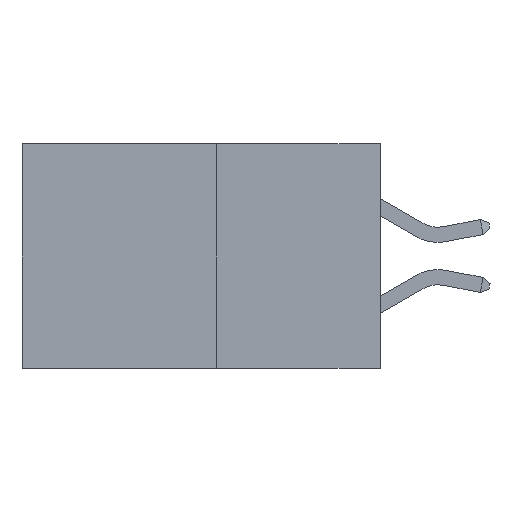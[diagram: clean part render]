
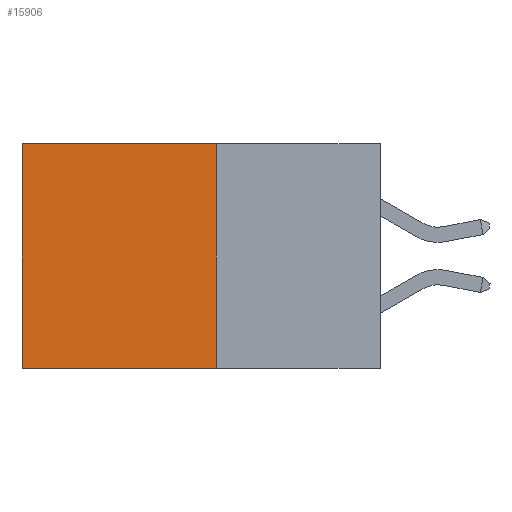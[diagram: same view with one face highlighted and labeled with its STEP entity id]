
A CAD part, left-side view. The second image highlights one B-rep face of the part: STEP entity #15906.
In plain terms, the highlighted planar face has unit normal (-1, 0, 0).
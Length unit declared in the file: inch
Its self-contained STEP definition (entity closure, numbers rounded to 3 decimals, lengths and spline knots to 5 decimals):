
#2518 = VECTOR ( 'NONE', #27617, 39.37008 ) ;
#2606 = CARTESIAN_POINT ( 'NONE',  ( 0.277, 0.59, -0.37 ) ) ;
#2663 = CARTESIAN_POINT ( 'NONE',  ( 0.277, 0.27, -0.37 ) ) ;
#2934 = EDGE_CURVE ( 'NONE', #24772, #28813, #3862, .T. ) ;
#3862 = LINE ( 'NONE', #2606, #9939 ) ;
#4960 = DIRECTION ( 'NONE',  ( 0., 0., -1. ) ) ;
#5658 = PLANE ( 'NONE',  #28293 ) ;
#6114 = VERTEX_POINT ( 'NONE', #24021 ) ;
#7324 = EDGE_CURVE ( 'NONE', #12484, #24772, #19964, .T. ) ;
#9293 = CARTESIAN_POINT ( 'NONE',  ( 0.277, 0.59, 0. ) ) ;
#9557 = CARTESIAN_POINT ( 'NONE',  ( 0.277, 0.27, -0.37 ) ) ;
#9939 = VECTOR ( 'NONE', #20922, 39.37008 ) ;
#10618 = LINE ( 'NONE', #2663, #27220 ) ;
#12484 = VERTEX_POINT ( 'NONE', #18467 ) ;
#13744 = CARTESIAN_POINT ( 'NONE',  ( 0.277, 0.59, -0.37 ) ) ;
#13921 = VECTOR ( 'NONE', #27863, 39.37008 ) ;
#14792 = DIRECTION ( 'NONE',  ( 0., 0., -1. ) ) ;
#15906 = ADVANCED_FACE ( 'NONE', ( #27357 ), #5658, .F. ) ;
#16366 = EDGE_CURVE ( 'NONE', #6114, #28813, #20688, .T. ) ;
#17384 = EDGE_LOOP ( 'NONE', ( #18318, #20697, #19676, #24008 ) ) ;
#18318 = ORIENTED_EDGE ( 'NONE', *, *, #2934, .T. ) ;
#18467 = CARTESIAN_POINT ( 'NONE',  ( 0.277, 0.27, 0. ) ) ;
#19291 = CARTESIAN_POINT ( 'NONE',  ( 0.277, 0.27, -0.37 ) ) ;
#19676 = ORIENTED_EDGE ( 'NONE', *, *, #21916, .F. ) ;
#19964 = LINE ( 'NONE', #25606, #13921 ) ;
#20688 = LINE ( 'NONE', #9557, #2518 ) ;
#20697 = ORIENTED_EDGE ( 'NONE', *, *, #16366, .F. ) ;
#20922 = DIRECTION ( 'NONE',  ( 0., 0., -1. ) ) ;
#21916 = EDGE_CURVE ( 'NONE', #12484, #6114, #10618, .T. ) ;
#24008 = ORIENTED_EDGE ( 'NONE', *, *, #7324, .T. ) ;
#24021 = CARTESIAN_POINT ( 'NONE',  ( 0.277, 0.27, -0.37 ) ) ;
#24772 = VERTEX_POINT ( 'NONE', #9293 ) ;
#25606 = CARTESIAN_POINT ( 'NONE',  ( 0.277, 0.27, 0. ) ) ;
#27220 = VECTOR ( 'NONE', #4960, 39.37008 ) ;
#27357 = FACE_OUTER_BOUND ( 'NONE', #17384, .T. ) ;
#27617 = DIRECTION ( 'NONE',  ( 0., 1., 0. ) ) ;
#27863 = DIRECTION ( 'NONE',  ( 0., 1., 0. ) ) ;
#28293 = AXIS2_PLACEMENT_3D ( 'NONE', #19291, #28313, #14792 ) ;
#28313 = DIRECTION ( 'NONE',  ( 1., 0., 0. ) ) ;
#28813 = VERTEX_POINT ( 'NONE', #13744 ) ;
